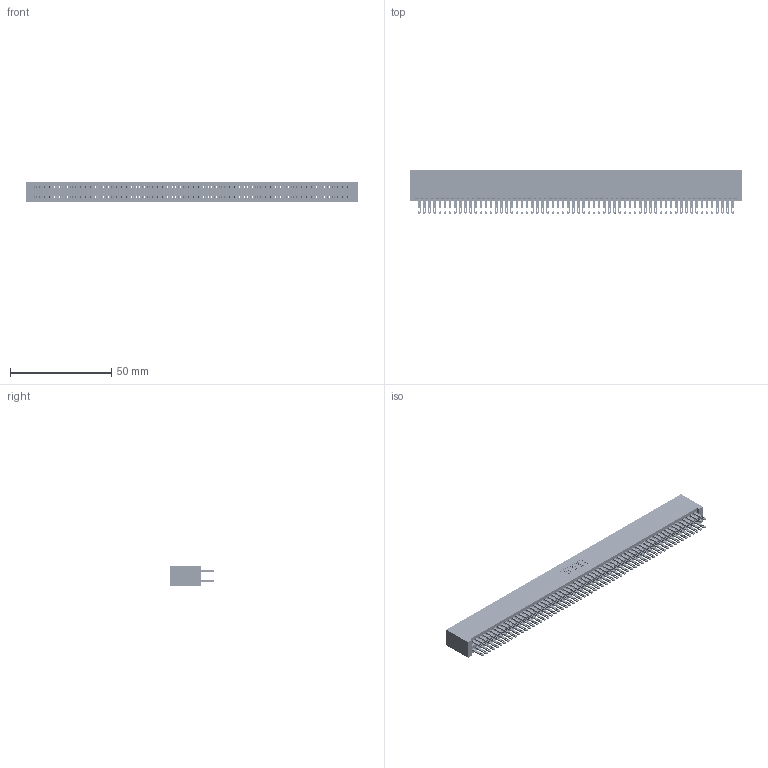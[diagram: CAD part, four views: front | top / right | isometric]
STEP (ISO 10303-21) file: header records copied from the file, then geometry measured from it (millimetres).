
FILE_DESCRIPTION (( 'STEP AP203' ), '1' );
FILE_NAME ('845-124-500-201.STEP', '2018-11-21T15:50:01', ( '' ), ( '' ), 'SwSTEP 2.0', 'SolidWorks 2016', '' );
FILE_SCHEMA (( 'CONFIG_CONTROL_DESIGN' ));
Length unit declared in the file: inch
Products named in the file (3): 845 Part_No Mounting Lugs; 345-292-001_345-293-100; 845-124-500-201
Assembly tree (125 placements, depth 2):
  845-124-500-201
    845 Part_No Mounting Lugs
    345-292-001_345-293-100  x124
Bounding box: 164.08 x 21.51 x 9.4 mm (x, y, z)
Volume: 17119.8 mm3; surface area: 27261.2 mm2
Topology: 125 solids, 125 shells, 5822 faces, 17801 edges, 11866 vertices
Faces by surface type: plane 3424, cylinder 2398
Entity records: 45607 total; most frequent: CARTESIAN_POINT 7624, ORIENTED_EDGE 7558, DIRECTION 6695, EDGE_CURVE 3779, LINE 3403, VECTOR 3403, VERTEX_POINT 2518, AXIS2_PLACEMENT_3D 1646
